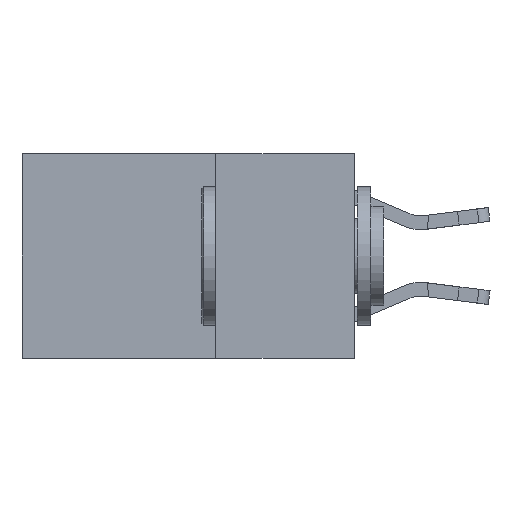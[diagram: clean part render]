
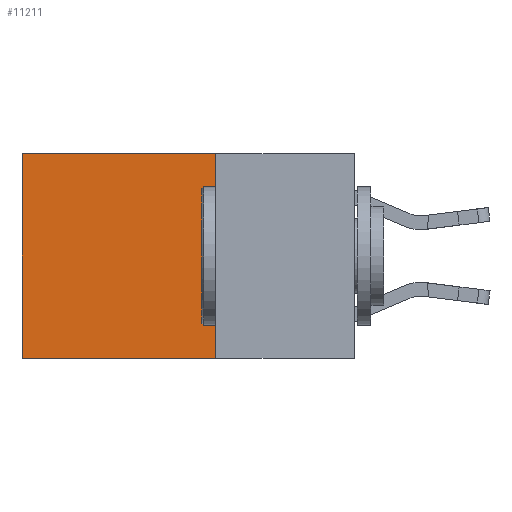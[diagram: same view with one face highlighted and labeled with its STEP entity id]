
A CAD part, left-side view. The second image highlights one B-rep face of the part: STEP entity #11211.
In plain terms, the highlighted planar face has unit normal (-1, 0, 0).
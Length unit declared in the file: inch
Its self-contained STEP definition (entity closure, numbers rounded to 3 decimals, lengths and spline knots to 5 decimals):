
#206 = VECTOR ( 'NONE', #9249, 39.37008 ) ;
#610 = CARTESIAN_POINT ( 'NONE',  ( 0.2625, 0.25, 0. ) ) ;
#1662 = DIRECTION ( 'NONE',  ( 0., 1., 0. ) ) ;
#2292 = FACE_OUTER_BOUND ( 'NONE', #9045, .T. ) ;
#2994 = ORIENTED_EDGE ( 'NONE', *, *, #12583, .T. ) ;
#3010 = CARTESIAN_POINT ( 'NONE',  ( 0.2625, 0.25, -0.37 ) ) ;
#3336 = ORIENTED_EDGE ( 'NONE', *, *, #6397, .F. ) ;
#3553 = CARTESIAN_POINT ( 'NONE',  ( 0.2625, 0.6, 0. ) ) ;
#3604 = CARTESIAN_POINT ( 'NONE',  ( 0.2625, 0.25, 0. ) ) ;
#3656 = CARTESIAN_POINT ( 'NONE',  ( 0.2625, 0.25, 0. ) ) ;
#4752 = VERTEX_POINT ( 'NONE', #3553 ) ;
#4781 = VECTOR ( 'NONE', #8913, 39.37008 ) ;
#5449 = DIRECTION ( 'NONE',  ( 0., 0., -1. ) ) ;
#5981 = EDGE_CURVE ( 'NONE', #6658, #7164, #13642, .T. ) ;
#6397 = EDGE_CURVE ( 'NONE', #11476, #6658, #12156, .T. ) ;
#6658 = VERTEX_POINT ( 'NONE', #9557 ) ;
#6898 = AXIS2_PLACEMENT_3D ( 'NONE', #13756, #7557, #5449 ) ;
#7164 = VERTEX_POINT ( 'NONE', #9146 ) ;
#7557 = DIRECTION ( 'NONE',  ( 1., 0., 0. ) ) ;
#8005 = LINE ( 'NONE', #3604, #12959 ) ;
#8126 = LINE ( 'NONE', #9975, #4781 ) ;
#8759 = PLANE ( 'NONE',  #6898 ) ;
#8913 = DIRECTION ( 'NONE',  ( 0., 0., -1. ) ) ;
#9045 = EDGE_LOOP ( 'NONE', ( #2994, #13470, #3336, #11144 ) ) ;
#9146 = CARTESIAN_POINT ( 'NONE',  ( 0.2625, 0.6, -0.37 ) ) ;
#9249 = DIRECTION ( 'NONE',  ( 0., 1., 0. ) ) ;
#9557 = CARTESIAN_POINT ( 'NONE',  ( 0.2625, 0.25, -0.37 ) ) ;
#9975 = CARTESIAN_POINT ( 'NONE',  ( 0.2625, 0.6, 0. ) ) ;
#10459 = EDGE_CURVE ( 'NONE', #11476, #4752, #8005, .T. ) ;
#11043 = DIRECTION ( 'NONE',  ( 0., 0., -1. ) ) ;
#11144 = ORIENTED_EDGE ( 'NONE', *, *, #10459, .T. ) ;
#11211 = ADVANCED_FACE ( 'NONE', ( #2292 ), #8759, .F. ) ;
#11476 = VERTEX_POINT ( 'NONE', #610 ) ;
#12156 = LINE ( 'NONE', #3656, #12482 ) ;
#12482 = VECTOR ( 'NONE', #11043, 39.37008 ) ;
#12583 = EDGE_CURVE ( 'NONE', #4752, #7164, #8126, .T. ) ;
#12959 = VECTOR ( 'NONE', #1662, 39.37008 ) ;
#13470 = ORIENTED_EDGE ( 'NONE', *, *, #5981, .F. ) ;
#13642 = LINE ( 'NONE', #3010, #206 ) ;
#13756 = CARTESIAN_POINT ( 'NONE',  ( 0.2625, 0.25, 0. ) ) ;
